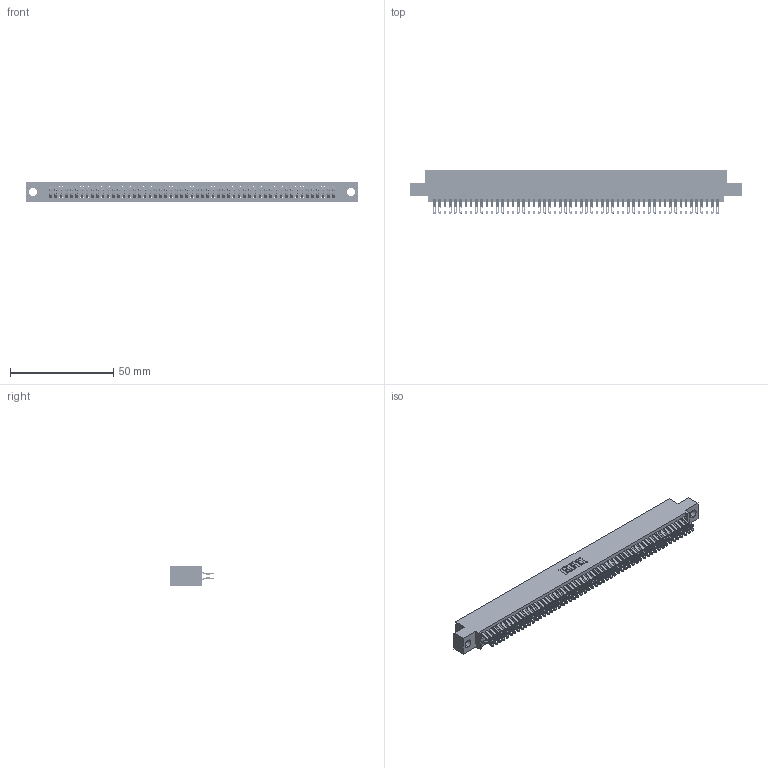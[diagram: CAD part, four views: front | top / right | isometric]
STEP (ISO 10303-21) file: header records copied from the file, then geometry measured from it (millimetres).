
FILE_DESCRIPTION (( 'STEP AP203' ), '1' );
FILE_NAME ('345-110-555-504.STEP', '2018-10-07T11:36:16', ( '' ), ( '' ), 'SwSTEP 2.0', 'SolidWorks 2016', '' );
FILE_SCHEMA (( 'CONFIG_CONTROL_DESIGN' ));
Length unit declared in the file: inch
Products named in the file (3): 345-292-001_555 Tail; 345 Part_0.110 Offset - 0.156 Dia-TH; 345-110-555-504
Assembly tree (111 placements, depth 2):
  345-110-555-504
    345 Part_0.110 Offset - 0.156 Dia-TH
    345-292-001_555 Tail  x110
Bounding box: 160.91 x 21.13 x 9.4 mm (x, y, z)
Volume: 15909.4 mm3; surface area: 24786.2 mm2
Topology: 111 solids, 111 shells, 6290 faces, 19823 edges, 13214 vertices
Faces by surface type: plane 3494, cylinder 2796
Entity records: 41865 total; most frequent: CARTESIAN_POINT 7042, ORIENTED_EDGE 6946, DIRECTION 6161, EDGE_CURVE 3473, LINE 3101, VECTOR 3101, VERTEX_POINT 2314, AXIS2_PLACEMENT_3D 1530
